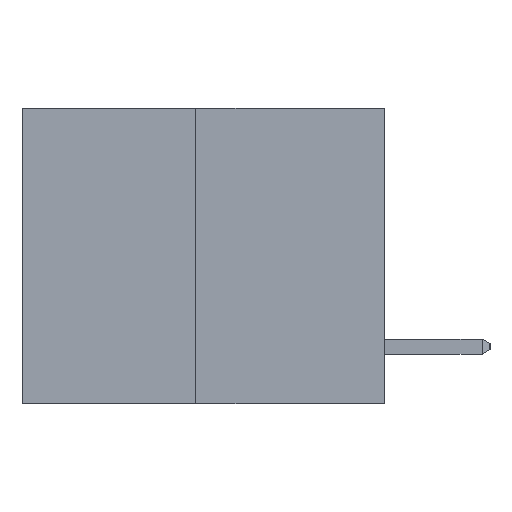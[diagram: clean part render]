
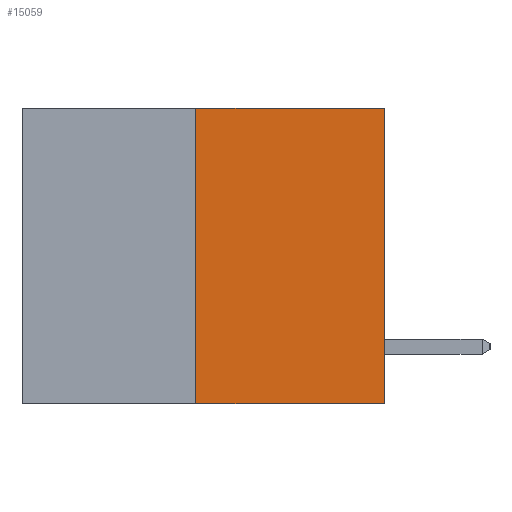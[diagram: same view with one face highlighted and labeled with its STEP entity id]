
A CAD part, left-side view. The second image highlights one B-rep face of the part: STEP entity #15059.
In plain terms, the highlighted planar face has unit normal (-1, 0, 0).
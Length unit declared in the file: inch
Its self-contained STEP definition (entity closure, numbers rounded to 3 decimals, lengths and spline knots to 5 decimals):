
#247 = EDGE_LOOP ( 'NONE', ( #15001, #19745, #10236, #691 ) ) ;
#263 = FACE_OUTER_BOUND ( 'NONE', #247, .T. ) ;
#550 = EDGE_CURVE ( 'NONE', #6492, #10972, #9096, .T. ) ;
#691 = ORIENTED_EDGE ( 'NONE', *, *, #4670, .F. ) ;
#1364 = PLANE ( 'NONE',  #9068 ) ;
#1502 = DIRECTION ( 'NONE',  ( 0., 0., 1. ) ) ;
#1582 = LINE ( 'NONE', #4341, #10017 ) ;
#2894 = CARTESIAN_POINT ( 'NONE',  ( 0., 0.312, -0.49 ) ) ;
#3321 = EDGE_CURVE ( 'NONE', #10972, #4812, #19968, .T. ) ;
#4030 = CARTESIAN_POINT ( 'NONE',  ( 0., 0., 0. ) ) ;
#4133 = DIRECTION ( 'NONE',  ( 0., -1., 0. ) ) ;
#4341 = CARTESIAN_POINT ( 'NONE',  ( 0., 0.312, -0.49 ) ) ;
#4358 = DIRECTION ( 'NONE',  ( 1., 0., 0. ) ) ;
#4670 = EDGE_CURVE ( 'NONE', #15372, #4812, #14882, .T. ) ;
#4812 = VERTEX_POINT ( 'NONE', #4030 ) ;
#4881 = VECTOR ( 'NONE', #4133, 39.37008 ) ;
#6350 = CARTESIAN_POINT ( 'NONE',  ( 0., 0.312, 0. ) ) ;
#6492 = VERTEX_POINT ( 'NONE', #2894 ) ;
#7237 = DIRECTION ( 'NONE',  ( 0., -1., 0. ) ) ;
#7944 = CARTESIAN_POINT ( 'NONE',  ( 0., 0., 0. ) ) ;
#9068 = AXIS2_PLACEMENT_3D ( 'NONE', #14069, #4358, #15670 ) ;
#9096 = LINE ( 'NONE', #18467, #4881 ) ;
#9119 = DIRECTION ( 'NONE',  ( 0., 0., 1. ) ) ;
#9896 = VECTOR ( 'NONE', #7237, 39.37008 ) ;
#10017 = VECTOR ( 'NONE', #9119, 39.37008 ) ;
#10236 = ORIENTED_EDGE ( 'NONE', *, *, #3321, .T. ) ;
#10972 = VERTEX_POINT ( 'NONE', #19259 ) ;
#14069 = CARTESIAN_POINT ( 'NONE',  ( 0., 0.6, 0. ) ) ;
#14882 = LINE ( 'NONE', #18658, #9896 ) ;
#15001 = ORIENTED_EDGE ( 'NONE', *, *, #19606, .F. ) ;
#15059 = ADVANCED_FACE ( 'NONE', ( #263 ), #1364, .F. ) ;
#15372 = VERTEX_POINT ( 'NONE', #6350 ) ;
#15670 = DIRECTION ( 'NONE',  ( 0., 0., -1. ) ) ;
#16721 = VECTOR ( 'NONE', #1502, 39.37008 ) ;
#18467 = CARTESIAN_POINT ( 'NONE',  ( 0., 0.6, -0.49 ) ) ;
#18658 = CARTESIAN_POINT ( 'NONE',  ( 0., 0.6, 0. ) ) ;
#19259 = CARTESIAN_POINT ( 'NONE',  ( 0., 0., -0.49 ) ) ;
#19606 = EDGE_CURVE ( 'NONE', #6492, #15372, #1582, .T. ) ;
#19745 = ORIENTED_EDGE ( 'NONE', *, *, #550, .T. ) ;
#19968 = LINE ( 'NONE', #7944, #16721 ) ;
